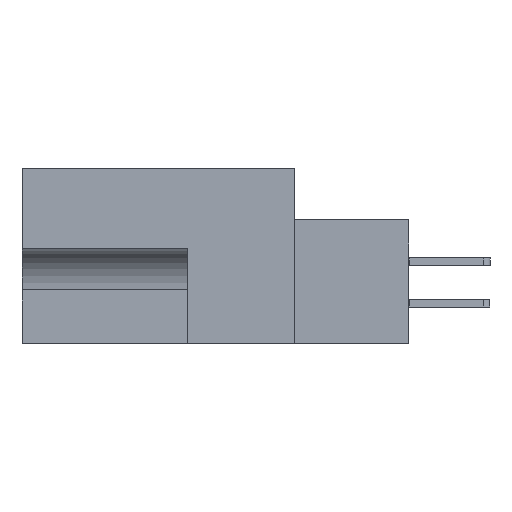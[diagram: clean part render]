
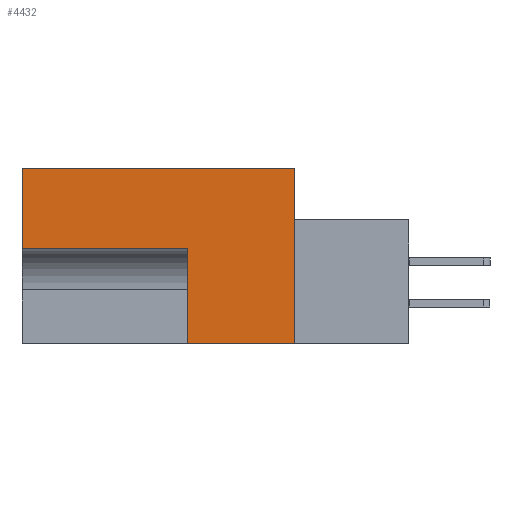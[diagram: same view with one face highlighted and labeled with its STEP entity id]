
A CAD part, left-side view. The second image highlights one B-rep face of the part: STEP entity #4432.
In plain terms, the highlighted planar face has unit normal (-1, 0, 0).
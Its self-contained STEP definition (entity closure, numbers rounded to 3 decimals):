
#608 = ORIENTED_EDGE ( 'NONE', *, *, #12918, .F. ) ;
#1366 = VECTOR ( 'NONE', #9721, 1000. ) ;
#1755 = DIRECTION ( 'NONE',  ( 0., 0., 1. ) ) ;
#3258 = LINE ( 'NONE', #31055, #11799 ) ;
#3345 = CARTESIAN_POINT ( 'NONE',  ( 0., 8.255, -13.487 ) ) ;
#4345 = CARTESIAN_POINT ( 'NONE',  ( 0., 20.955, -13.487 ) ) ;
#4432 = ADVANCED_FACE ( 'NONE', ( #7261 ), #6359, .F. ) ;
#5758 = CARTESIAN_POINT ( 'NONE',  ( 0., 11.506, 0. ) ) ;
#6359 = PLANE ( 'NONE',  #30559 ) ;
#7261 = FACE_OUTER_BOUND ( 'NONE', #9969, .T. ) ;
#7766 = LINE ( 'NONE', #5758, #15455 ) ;
#7818 = VERTEX_POINT ( 'NONE', #9471 ) ;
#8795 = ORIENTED_EDGE ( 'NONE', *, *, #19910, .F. ) ;
#9471 = CARTESIAN_POINT ( 'NONE',  ( 0., 0., -13.487 ) ) ;
#9721 = DIRECTION ( 'NONE',  ( 0., 0., 1. ) ) ;
#9953 = CARTESIAN_POINT ( 'NONE',  ( 0., 20.955, 0. ) ) ;
#9969 = EDGE_LOOP ( 'NONE', ( #608, #8795, #17757, #22064, #33914, #12723 ) ) ;
#10795 = VECTOR ( 'NONE', #1755, 1000. ) ;
#11647 = DIRECTION ( 'NONE',  ( 0., -1., 0. ) ) ;
#11799 = VECTOR ( 'NONE', #11915, 1000. ) ;
#11883 = DIRECTION ( 'NONE',  ( 0., 0., -1. ) ) ;
#11915 = DIRECTION ( 'NONE',  ( 0., 1., 0. ) ) ;
#12723 = ORIENTED_EDGE ( 'NONE', *, *, #23183, .F. ) ;
#12918 = EDGE_CURVE ( 'NONE', #7818, #17654, #3258, .T. ) ;
#13737 = VERTEX_POINT ( 'NONE', #9953 ) ;
#15455 = VECTOR ( 'NONE', #11647, 1000. ) ;
#17654 = VERTEX_POINT ( 'NONE', #3345 ) ;
#17757 = ORIENTED_EDGE ( 'NONE', *, *, #23491, .F. ) ;
#17899 = VERTEX_POINT ( 'NONE', #35424 ) ;
#18325 = CARTESIAN_POINT ( 'NONE',  ( 0., 0., 0. ) ) ;
#18743 = VECTOR ( 'NONE', #21080, 1000. ) ;
#19910 = EDGE_CURVE ( 'NONE', #17899, #7818, #21314, .T. ) ;
#20250 = DIRECTION ( 'NONE',  ( 1., 0., 0. ) ) ;
#21080 = DIRECTION ( 'NONE',  ( 0., 0., -1. ) ) ;
#21314 = LINE ( 'NONE', #18325, #18743 ) ;
#22064 = ORIENTED_EDGE ( 'NONE', *, *, #23608, .F. ) ;
#23183 = EDGE_CURVE ( 'NONE', #17654, #34549, #33903, .T. ) ;
#23252 = CARTESIAN_POINT ( 'NONE',  ( 0., 8.255, -6.172 ) ) ;
#23491 = EDGE_CURVE ( 'NONE', #13737, #17899, #7766, .T. ) ;
#23608 = EDGE_CURVE ( 'NONE', #30276, #13737, #30875, .T. ) ;
#23889 = CARTESIAN_POINT ( 'NONE',  ( 0., 8.255, -13.487 ) ) ;
#24187 = CARTESIAN_POINT ( 'NONE',  ( 0., 20.955, -6.172 ) ) ;
#24466 = EDGE_CURVE ( 'NONE', #34549, #30276, #29933, .T. ) ;
#25564 = CARTESIAN_POINT ( 'NONE',  ( 0., 0., 0. ) ) ;
#28071 = CARTESIAN_POINT ( 'NONE',  ( 0., 8.255, -6.172 ) ) ;
#28227 = VECTOR ( 'NONE', #28425, 1000. ) ;
#28425 = DIRECTION ( 'NONE',  ( 0., 1., 0. ) ) ;
#29933 = LINE ( 'NONE', #28071, #28227 ) ;
#30276 = VERTEX_POINT ( 'NONE', #24187 ) ;
#30559 = AXIS2_PLACEMENT_3D ( 'NONE', #25564, #20250, #11883 ) ;
#30875 = LINE ( 'NONE', #4345, #1366 ) ;
#31055 = CARTESIAN_POINT ( 'NONE',  ( 0., -8.814, -13.487 ) ) ;
#33903 = LINE ( 'NONE', #23889, #10795 ) ;
#33914 = ORIENTED_EDGE ( 'NONE', *, *, #24466, .F. ) ;
#34549 = VERTEX_POINT ( 'NONE', #23252 ) ;
#35424 = CARTESIAN_POINT ( 'NONE',  ( 0., 0., 0. ) ) ;
